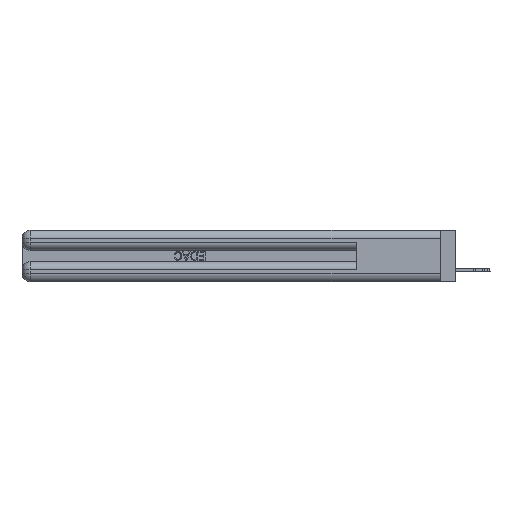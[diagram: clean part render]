
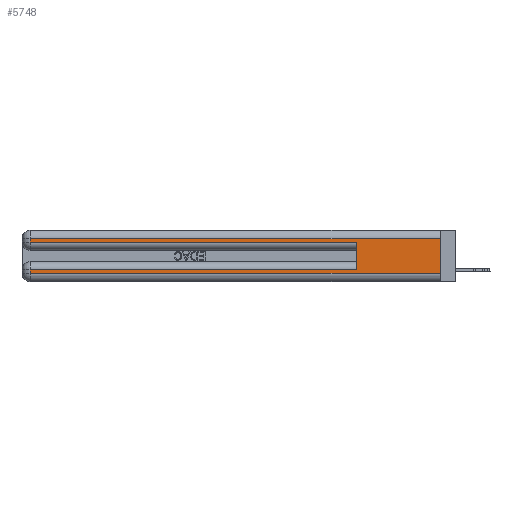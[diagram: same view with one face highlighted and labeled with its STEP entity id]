
A CAD part, left-side view. The second image highlights one B-rep face of the part: STEP entity #5748.
In plain terms, the highlighted planar face has unit normal (-1, 0, 0).
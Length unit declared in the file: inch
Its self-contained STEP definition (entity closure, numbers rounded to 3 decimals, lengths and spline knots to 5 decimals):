
#1080 = EDGE_CURVE ( 'NONE', #34942, #18649, #15443, .T. ) ;
#1361 = CARTESIAN_POINT ( 'NONE',  ( 0., 2.94, 0.31 ) ) ;
#4064 = FACE_OUTER_BOUND ( 'NONE', #27606, .T. ) ;
#4065 = ORIENTED_EDGE ( 'NONE', *, *, #20821, .T. ) ;
#4852 = VECTOR ( 'NONE', #31595, 39.37008 ) ;
#5592 = PLANE ( 'NONE',  #16524 ) ;
#5748 = ADVANCED_FACE ( 'NONE', ( #4064 ), #5592, .F. ) ;
#6970 = VECTOR ( 'NONE', #36855, 39.37008 ) ;
#7257 = DIRECTION ( 'NONE',  ( 0., -1., 0. ) ) ;
#8891 = DIRECTION ( 'NONE',  ( 1., 0., 0. ) ) ;
#9283 = DIRECTION ( 'NONE',  ( 0., 0., -1. ) ) ;
#9487 = EDGE_CURVE ( 'NONE', #34408, #12695, #13562, .T. ) ;
#10224 = ORIENTED_EDGE ( 'NONE', *, *, #1080, .T. ) ;
#10803 = CARTESIAN_POINT ( 'NONE',  ( 0., 0.6, 0.085 ) ) ;
#12031 = DIRECTION ( 'NONE',  ( 0., 1., 0. ) ) ;
#12189 = ORIENTED_EDGE ( 'NONE', *, *, #9487, .T. ) ;
#12261 = DIRECTION ( 'NONE',  ( 0., 0., 1. ) ) ;
#12473 = LINE ( 'NONE', #39993, #34814 ) ;
#12695 = VERTEX_POINT ( 'NONE', #16599 ) ;
#12764 = LINE ( 'NONE', #27045, #22712 ) ;
#12971 = ORIENTED_EDGE ( 'NONE', *, *, #16797, .F. ) ;
#13258 = VERTEX_POINT ( 'NONE', #10803 ) ;
#13562 = LINE ( 'NONE', #17816, #29497 ) ;
#13662 = VECTOR ( 'NONE', #12261, 39.37008 ) ;
#14683 = CARTESIAN_POINT ( 'NONE',  ( 0., 2.94, 0.37 ) ) ;
#15153 = CARTESIAN_POINT ( 'NONE',  ( 0., 0., 0.37 ) ) ;
#15443 = LINE ( 'NONE', #14683, #6970 ) ;
#15957 = VERTEX_POINT ( 'NONE', #19319 ) ;
#16524 = AXIS2_PLACEMENT_3D ( 'NONE', #15153, #8891, #9283 ) ;
#16599 = CARTESIAN_POINT ( 'NONE',  ( 0., 0., 0.06 ) ) ;
#16797 = EDGE_CURVE ( 'NONE', #13258, #15957, #38016, .T. ) ;
#16891 = LINE ( 'NONE', #21230, #24416 ) ;
#17816 = CARTESIAN_POINT ( 'NONE',  ( 0., 0., 0.06 ) ) ;
#18649 = VERTEX_POINT ( 'NONE', #26492 ) ;
#19319 = CARTESIAN_POINT ( 'NONE',  ( 0., 0.6, 0.285 ) ) ;
#19825 = EDGE_CURVE ( 'NONE', #13258, #32309, #16891, .T. ) ;
#20332 = LINE ( 'NONE', #26155, #27794 ) ;
#20430 = DIRECTION ( 'NONE',  ( 0., 0., -1. ) ) ;
#20821 = EDGE_CURVE ( 'NONE', #18649, #15957, #20332, .T. ) ;
#21230 = CARTESIAN_POINT ( 'NONE',  ( 0., 0., 0.085 ) ) ;
#22253 = VERTEX_POINT ( 'NONE', #38310 ) ;
#22712 = VECTOR ( 'NONE', #30219, 39.37008 ) ;
#23538 = DIRECTION ( 'NONE',  ( 0., -1., 0. ) ) ;
#24416 = VECTOR ( 'NONE', #12031, 39.37008 ) ;
#25401 = ORIENTED_EDGE ( 'NONE', *, *, #36886, .F. ) ;
#26051 = CARTESIAN_POINT ( 'NONE',  ( 0., 2.94, 0.085 ) ) ;
#26155 = CARTESIAN_POINT ( 'NONE',  ( 0., 0., 0.285 ) ) ;
#26492 = CARTESIAN_POINT ( 'NONE',  ( 0., 2.94, 0.285 ) ) ;
#27045 = CARTESIAN_POINT ( 'NONE',  ( 0., 2.94, 0.37 ) ) ;
#27606 = EDGE_LOOP ( 'NONE', ( #25401, #27890, #10224, #4065, #12971, #28518, #28017, #12189 ) ) ;
#27794 = VECTOR ( 'NONE', #7257, 39.37008 ) ;
#27890 = ORIENTED_EDGE ( 'NONE', *, *, #29848, .T. ) ;
#28017 = ORIENTED_EDGE ( 'NONE', *, *, #37451, .T. ) ;
#28431 = CARTESIAN_POINT ( 'NONE',  ( 0., 0., 0.31 ) ) ;
#28518 = ORIENTED_EDGE ( 'NONE', *, *, #19825, .T. ) ;
#28672 = LINE ( 'NONE', #28431, #4852 ) ;
#29457 = CARTESIAN_POINT ( 'NONE',  ( 0., 2.94, 0.06 ) ) ;
#29497 = VECTOR ( 'NONE', #23538, 39.37008 ) ;
#29848 = EDGE_CURVE ( 'NONE', #22253, #34942, #28672, .T. ) ;
#30219 = DIRECTION ( 'NONE',  ( 0., 0., -1. ) ) ;
#31422 = CARTESIAN_POINT ( 'NONE',  ( 0., 0.6, 0.145 ) ) ;
#31595 = DIRECTION ( 'NONE',  ( 0., 1., 0. ) ) ;
#32309 = VERTEX_POINT ( 'NONE', #26051 ) ;
#34408 = VERTEX_POINT ( 'NONE', #29457 ) ;
#34814 = VECTOR ( 'NONE', #20430, 39.37008 ) ;
#34942 = VERTEX_POINT ( 'NONE', #1361 ) ;
#36855 = DIRECTION ( 'NONE',  ( 0., 0., -1. ) ) ;
#36886 = EDGE_CURVE ( 'NONE', #22253, #12695, #12473, .T. ) ;
#37451 = EDGE_CURVE ( 'NONE', #32309, #34408, #12764, .T. ) ;
#38016 = LINE ( 'NONE', #31422, #13662 ) ;
#38310 = CARTESIAN_POINT ( 'NONE',  ( 0., 0., 0.31 ) ) ;
#39993 = CARTESIAN_POINT ( 'NONE',  ( 0., 0., 0.37 ) ) ;
